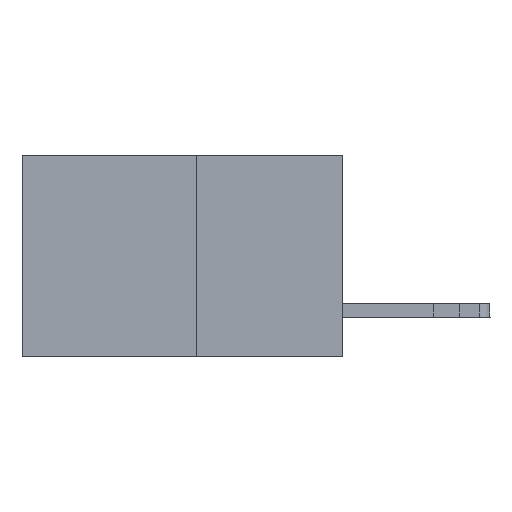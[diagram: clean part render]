
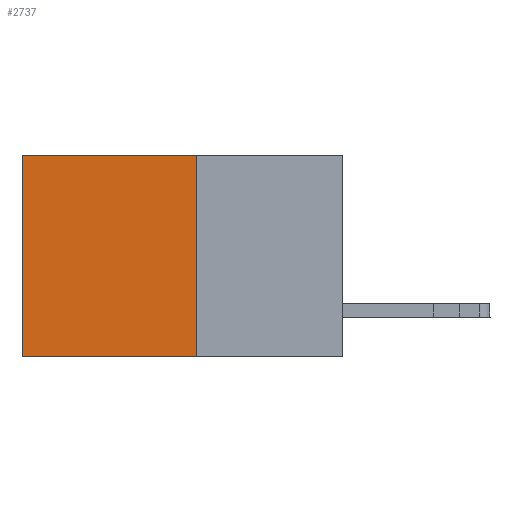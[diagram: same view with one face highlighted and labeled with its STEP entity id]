
A CAD part, left-side view. The second image highlights one B-rep face of the part: STEP entity #2737.
In plain terms, the highlighted planar face has unit normal (-1, 0, 0).
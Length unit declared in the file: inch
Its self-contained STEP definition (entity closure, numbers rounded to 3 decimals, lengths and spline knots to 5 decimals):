
#64 = EDGE_CURVE ( 'NONE', #8937, #6427, #15601, .T. ) ;
#98 = PLANE ( 'NONE',  #2301 ) ;
#514 = EDGE_CURVE ( 'NONE', #6427, #16403, #12850, .T. ) ;
#938 = ORIENTED_EDGE ( 'NONE', *, *, #514, .T. ) ;
#1484 = VECTOR ( 'NONE', #7109, 39.37008 ) ;
#2301 = AXIS2_PLACEMENT_3D ( 'NONE', #11169, #10047, #11438 ) ;
#2737 = ADVANCED_FACE ( 'NONE', ( #14060 ), #98, .F. ) ;
#3101 = CARTESIAN_POINT ( 'NONE',  ( 0.277, 0.27, 0. ) ) ;
#4614 = DIRECTION ( 'NONE',  ( 0., 1., 0. ) ) ;
#5111 = ORIENTED_EDGE ( 'NONE', *, *, #13900, .F. ) ;
#5129 = CARTESIAN_POINT ( 'NONE',  ( 0.277, 0.27, 0. ) ) ;
#5556 = ORIENTED_EDGE ( 'NONE', *, *, #17014, .F. ) ;
#6427 = VERTEX_POINT ( 'NONE', #15312 ) ;
#6998 = CARTESIAN_POINT ( 'NONE',  ( 0.277, 0.59, -0.37 ) ) ;
#7109 = DIRECTION ( 'NONE',  ( 0., 1., 0. ) ) ;
#8098 = VECTOR ( 'NONE', #14999, 39.37008 ) ;
#8694 = VERTEX_POINT ( 'NONE', #17422 ) ;
#8937 = VERTEX_POINT ( 'NONE', #5129 ) ;
#9308 = CARTESIAN_POINT ( 'NONE',  ( 0.277, 0.27, -0.37 ) ) ;
#10047 = DIRECTION ( 'NONE',  ( 1., 0., 0. ) ) ;
#11169 = CARTESIAN_POINT ( 'NONE',  ( 0.277, 0.27, -0.37 ) ) ;
#11438 = DIRECTION ( 'NONE',  ( 0., 0., -1. ) ) ;
#11461 = DIRECTION ( 'NONE',  ( 0., 0., -1. ) ) ;
#11774 = CARTESIAN_POINT ( 'NONE',  ( 0.277, 0.27, -0.37 ) ) ;
#12850 = LINE ( 'NONE', #6998, #17533 ) ;
#13225 = VECTOR ( 'NONE', #4614, 39.37008 ) ;
#13682 = ORIENTED_EDGE ( 'NONE', *, *, #64, .T. ) ;
#13900 = EDGE_CURVE ( 'NONE', #8937, #8694, #16399, .T. ) ;
#14060 = FACE_OUTER_BOUND ( 'NONE', #14890, .T. ) ;
#14890 = EDGE_LOOP ( 'NONE', ( #938, #5556, #5111, #13682 ) ) ;
#14999 = DIRECTION ( 'NONE',  ( 0., 0., -1. ) ) ;
#15312 = CARTESIAN_POINT ( 'NONE',  ( 0.277, 0.59, 0. ) ) ;
#15601 = LINE ( 'NONE', #3101, #1484 ) ;
#16172 = LINE ( 'NONE', #11774, #13225 ) ;
#16399 = LINE ( 'NONE', #9308, #8098 ) ;
#16403 = VERTEX_POINT ( 'NONE', #18192 ) ;
#17014 = EDGE_CURVE ( 'NONE', #8694, #16403, #16172, .T. ) ;
#17422 = CARTESIAN_POINT ( 'NONE',  ( 0.277, 0.27, -0.37 ) ) ;
#17533 = VECTOR ( 'NONE', #11461, 39.37008 ) ;
#18192 = CARTESIAN_POINT ( 'NONE',  ( 0.277, 0.59, -0.37 ) ) ;
